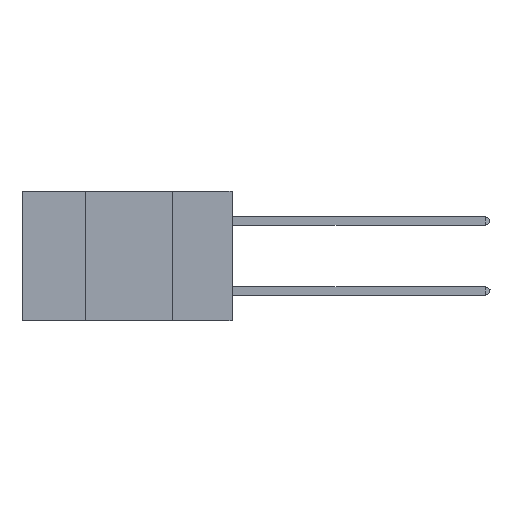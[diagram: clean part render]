
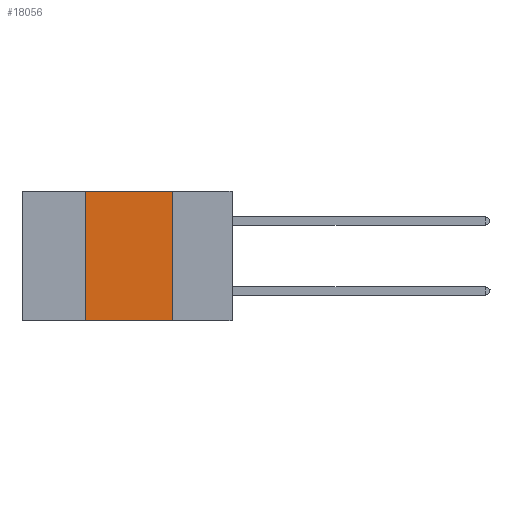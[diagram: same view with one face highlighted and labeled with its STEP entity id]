
A CAD part, left-side view. The second image highlights one B-rep face of the part: STEP entity #18056.
In plain terms, the highlighted planar face has unit normal (-1, 0, 0).
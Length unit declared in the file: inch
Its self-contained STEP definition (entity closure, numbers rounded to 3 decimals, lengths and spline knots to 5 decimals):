
#188 = CARTESIAN_POINT ( 'NONE',  ( 0., 0.17, 0. ) ) ;
#398 = CARTESIAN_POINT ( 'NONE',  ( 0., 0.42, 0. ) ) ;
#758 = VERTEX_POINT ( 'NONE', #188 ) ;
#833 = VERTEX_POINT ( 'NONE', #21637 ) ;
#1382 = EDGE_CURVE ( 'NONE', #758, #4298, #24562, .T. ) ;
#1498 = LINE ( 'NONE', #15897, #25236 ) ;
#4207 = CARTESIAN_POINT ( 'NONE',  ( 0., 0.17, -0.37 ) ) ;
#4298 = VERTEX_POINT ( 'NONE', #4207 ) ;
#4866 = DIRECTION ( 'NONE',  ( 0., 0., -1. ) ) ;
#5383 = VERTEX_POINT ( 'NONE', #398 ) ;
#5675 = VECTOR ( 'NONE', #22784, 39.37008 ) ;
#6907 = DIRECTION ( 'NONE',  ( 1., 0., 0. ) ) ;
#8018 = EDGE_LOOP ( 'NONE', ( #11261, #17594, #13980, #25518 ) ) ;
#9436 = PLANE ( 'NONE',  #13741 ) ;
#11261 = ORIENTED_EDGE ( 'NONE', *, *, #1382, .F. ) ;
#13741 = AXIS2_PLACEMENT_3D ( 'NONE', #17228, #6907, #4866 ) ;
#13980 = ORIENTED_EDGE ( 'NONE', *, *, #23325, .F. ) ;
#15196 = EDGE_CURVE ( 'NONE', #833, #4298, #24557, .T. ) ;
#15897 = CARTESIAN_POINT ( 'NONE',  ( 0., 0.6, 0. ) ) ;
#16034 = DIRECTION ( 'NONE',  ( 0., -1., 0. ) ) ;
#17228 = CARTESIAN_POINT ( 'NONE',  ( 0., 0.6, 0. ) ) ;
#17514 = CARTESIAN_POINT ( 'NONE',  ( 0., 0.17, 0. ) ) ;
#17594 = ORIENTED_EDGE ( 'NONE', *, *, #24504, .F. ) ;
#18056 = ADVANCED_FACE ( 'NONE', ( #25907 ), #9436, .F. ) ;
#18604 = CARTESIAN_POINT ( 'NONE',  ( 0., 0.42, 0. ) ) ;
#18879 = VECTOR ( 'NONE', #26456, 39.37008 ) ;
#19691 = DIRECTION ( 'NONE',  ( 0., 0., -1. ) ) ;
#20355 = CARTESIAN_POINT ( 'NONE',  ( 0., 0.6, -0.37 ) ) ;
#20631 = LINE ( 'NONE', #18604, #5675 ) ;
#21637 = CARTESIAN_POINT ( 'NONE',  ( 0., 0.42, -0.37 ) ) ;
#21821 = VECTOR ( 'NONE', #19691, 39.37008 ) ;
#22784 = DIRECTION ( 'NONE',  ( 0., 0., 1. ) ) ;
#23325 = EDGE_CURVE ( 'NONE', #833, #5383, #20631, .T. ) ;
#24504 = EDGE_CURVE ( 'NONE', #5383, #758, #1498, .T. ) ;
#24557 = LINE ( 'NONE', #20355, #18879 ) ;
#24562 = LINE ( 'NONE', #17514, #21821 ) ;
#25236 = VECTOR ( 'NONE', #16034, 39.37008 ) ;
#25518 = ORIENTED_EDGE ( 'NONE', *, *, #15196, .T. ) ;
#25907 = FACE_OUTER_BOUND ( 'NONE', #8018, .T. ) ;
#26456 = DIRECTION ( 'NONE',  ( 0., -1., 0. ) ) ;
